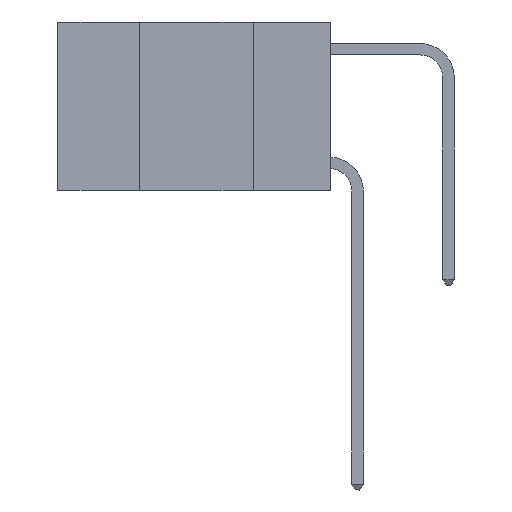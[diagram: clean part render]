
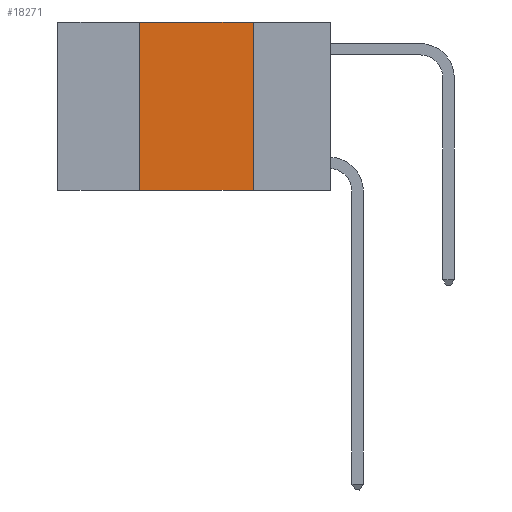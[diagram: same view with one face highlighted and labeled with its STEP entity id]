
A CAD part, left-side view. The second image highlights one B-rep face of the part: STEP entity #18271.
In plain terms, the highlighted planar face has unit normal (-1, 0, 0).
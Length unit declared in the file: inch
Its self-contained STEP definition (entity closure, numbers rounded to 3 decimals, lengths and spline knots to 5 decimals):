
#1299 = VECTOR ( 'NONE', #17178, 39.37008 ) ;
#2244 = DIRECTION ( 'NONE',  ( 0., 0., 1. ) ) ;
#3457 = AXIS2_PLACEMENT_3D ( 'NONE', #6969, #18040, #5226 ) ;
#4420 = ORIENTED_EDGE ( 'NONE', *, *, #10914, .F. ) ;
#4848 = EDGE_CURVE ( 'NONE', #13259, #5229, #10792, .T. ) ;
#5226 = DIRECTION ( 'NONE',  ( 0., 0., -1. ) ) ;
#5229 = VERTEX_POINT ( 'NONE', #19270 ) ;
#6586 = CARTESIAN_POINT ( 'NONE',  ( 0., 0.42, 0. ) ) ;
#6774 = FACE_OUTER_BOUND ( 'NONE', #12874, .T. ) ;
#6842 = CARTESIAN_POINT ( 'NONE',  ( 0., 0.42, 0. ) ) ;
#6969 = CARTESIAN_POINT ( 'NONE',  ( 0., 0.6, 0. ) ) ;
#8223 = ORIENTED_EDGE ( 'NONE', *, *, #18470, .T. ) ;
#9276 = CARTESIAN_POINT ( 'NONE',  ( 0., 0.6, 0. ) ) ;
#9626 = CARTESIAN_POINT ( 'NONE',  ( 0., 0.42, -0.37 ) ) ;
#9715 = LINE ( 'NONE', #16826, #1299 ) ;
#9819 = LINE ( 'NONE', #6842, #17061 ) ;
#10792 = LINE ( 'NONE', #18139, #12276 ) ;
#10914 = EDGE_CURVE ( 'NONE', #17182, #16071, #9819, .T. ) ;
#11635 = ORIENTED_EDGE ( 'NONE', *, *, #4848, .F. ) ;
#11697 = VECTOR ( 'NONE', #18598, 39.37008 ) ;
#12109 = ORIENTED_EDGE ( 'NONE', *, *, #18535, .F. ) ;
#12276 = VECTOR ( 'NONE', #13317, 39.37008 ) ;
#12874 = EDGE_LOOP ( 'NONE', ( #11635, #12109, #4420, #8223 ) ) ;
#13259 = VERTEX_POINT ( 'NONE', #17874 ) ;
#13317 = DIRECTION ( 'NONE',  ( 0., 0., -1. ) ) ;
#16071 = VERTEX_POINT ( 'NONE', #6586 ) ;
#16355 = PLANE ( 'NONE',  #3457 ) ;
#16826 = CARTESIAN_POINT ( 'NONE',  ( 0., 0.6, -0.37 ) ) ;
#17061 = VECTOR ( 'NONE', #2244, 39.37008 ) ;
#17178 = DIRECTION ( 'NONE',  ( 0., -1., 0. ) ) ;
#17182 = VERTEX_POINT ( 'NONE', #9626 ) ;
#17874 = CARTESIAN_POINT ( 'NONE',  ( 0., 0.17, 0. ) ) ;
#18040 = DIRECTION ( 'NONE',  ( 1., 0., 0. ) ) ;
#18139 = CARTESIAN_POINT ( 'NONE',  ( 0., 0.17, 0. ) ) ;
#18271 = ADVANCED_FACE ( 'NONE', ( #6774 ), #16355, .F. ) ;
#18470 = EDGE_CURVE ( 'NONE', #17182, #5229, #9715, .T. ) ;
#18535 = EDGE_CURVE ( 'NONE', #16071, #13259, #20133, .T. ) ;
#18598 = DIRECTION ( 'NONE',  ( 0., -1., 0. ) ) ;
#19270 = CARTESIAN_POINT ( 'NONE',  ( 0., 0.17, -0.37 ) ) ;
#20133 = LINE ( 'NONE', #9276, #11697 ) ;
